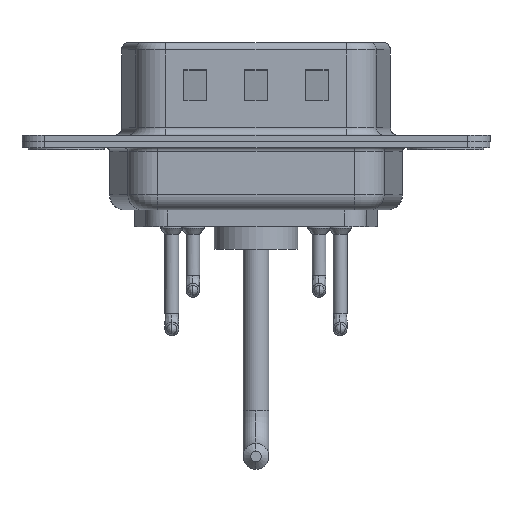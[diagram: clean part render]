
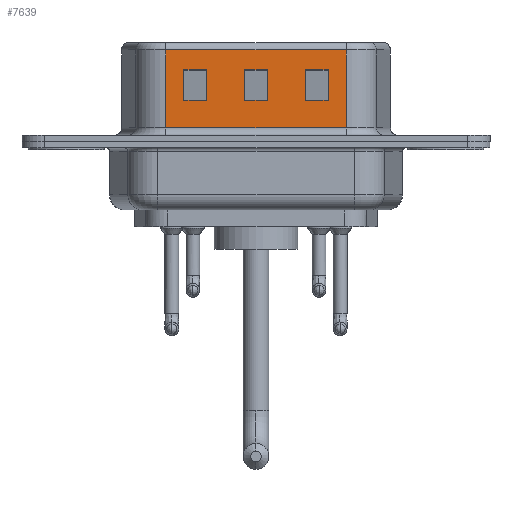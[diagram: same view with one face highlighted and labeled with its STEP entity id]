
A CAD part, front view. The second image highlights one B-rep face of the part: STEP entity #7639.
In plain terms, the highlighted planar face has unit normal (0, -1, 0).
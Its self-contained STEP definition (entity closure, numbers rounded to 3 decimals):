
#129 = ORIENTED_EDGE ( 'NONE', *, *, #16119, .T. ) ;
#251 = ORIENTED_EDGE ( 'NONE', *, *, #10598, .T. ) ;
#313 = CARTESIAN_POINT ( 'NONE',  ( 15.75, -4.55, 6.52 ) ) ;
#645 = VERTEX_POINT ( 'NONE', #16129 ) ;
#660 = CARTESIAN_POINT ( 'NONE',  ( 17.25, -4.55, 6.52 ) ) ;
#1310 = VERTEX_POINT ( 'NONE', #7896 ) ;
#1471 = DIRECTION ( 'NONE',  ( 1., 0., 0. ) ) ;
#1472 = EDGE_CURVE ( 'NONE', #3270, #1825, #12163, .T. ) ;
#1519 = LINE ( 'NONE', #12432, #11409 ) ;
#1825 = VERTEX_POINT ( 'NONE', #3703 ) ;
#1868 = VECTOR ( 'NONE', #4158, 1000. ) ;
#1922 = CARTESIAN_POINT ( 'NONE',  ( 18.451, -4.55, 6.02 ) ) ;
#2326 = VECTOR ( 'NONE', #16061, 1000. ) ;
#2384 = CARTESIAN_POINT ( 'NONE',  ( 7.75, -4.55, 4.705 ) ) ;
#2574 = CARTESIAN_POINT ( 'NONE',  ( 18.451, -4.55, 2.705 ) ) ;
#2583 = AXIS2_PLACEMENT_3D ( 'NONE', #14871, #13465, #9358 ) ;
#2734 = CARTESIAN_POINT ( 'NONE',  ( 9.25, -4.55, 6.52 ) ) ;
#2764 = DIRECTION ( 'NONE',  ( 0., 0., 1. ) ) ;
#3113 = DIRECTION ( 'NONE',  ( 1., 0., 0. ) ) ;
#3270 = VERTEX_POINT ( 'NONE', #14384 ) ;
#3328 = ORIENTED_EDGE ( 'NONE', *, *, #5694, .T. ) ;
#3396 = CARTESIAN_POINT ( 'NONE',  ( 7.75, -4.55, 6.52 ) ) ;
#3569 = VERTEX_POINT ( 'NONE', #11280 ) ;
#3645 = VECTOR ( 'NONE', #3113, 1000. ) ;
#3667 = LINE ( 'NONE', #11515, #8011 ) ;
#3675 = DIRECTION ( 'NONE',  ( 1., 0., 0. ) ) ;
#3703 = CARTESIAN_POINT ( 'NONE',  ( 6.549, -4.55, 0.9 ) ) ;
#3888 = VERTEX_POINT ( 'NONE', #16723 ) ;
#3982 = CARTESIAN_POINT ( 'NONE',  ( 6.549, -4.55, 6.52 ) ) ;
#4158 = DIRECTION ( 'NONE',  ( 0., 0., -1. ) ) ;
#4174 = EDGE_CURVE ( 'NONE', #8038, #3888, #8515, .T. ) ;
#4346 = VERTEX_POINT ( 'NONE', #6138 ) ;
#4417 = EDGE_LOOP ( 'NONE', ( #129, #14806, #17262, #14542 ) ) ;
#4756 = DIRECTION ( 'NONE',  ( 0., 0., -1. ) ) ;
#4987 = DIRECTION ( 'NONE',  ( -1., 0., 0. ) ) ;
#4997 = LINE ( 'NONE', #3396, #13685 ) ;
#5080 = CARTESIAN_POINT ( 'NONE',  ( 11.75, -4.55, 4.705 ) ) ;
#5178 = ORIENTED_EDGE ( 'NONE', *, *, #10489, .T. ) ;
#5450 = VERTEX_POINT ( 'NONE', #13937 ) ;
#5522 = VECTOR ( 'NONE', #15369, 1000. ) ;
#5602 = ORIENTED_EDGE ( 'NONE', *, *, #13185, .T. ) ;
#5694 = EDGE_CURVE ( 'NONE', #8637, #4346, #8235, .T. ) ;
#5772 = EDGE_CURVE ( 'NONE', #5450, #6888, #9490, .T. ) ;
#5799 = CARTESIAN_POINT ( 'NONE',  ( 18.451, -4.55, 4.705 ) ) ;
#6076 = DIRECTION ( 'NONE',  ( 0., 0., -1. ) ) ;
#6138 = CARTESIAN_POINT ( 'NONE',  ( 15.75, -4.55, 2.705 ) ) ;
#6238 = DIRECTION ( 'NONE',  ( 0., 0., 1. ) ) ;
#6563 = CARTESIAN_POINT ( 'NONE',  ( 18.451, -4.55, 6.02 ) ) ;
#6572 = DIRECTION ( 'NONE',  ( -1., 0., 0. ) ) ;
#6747 = DIRECTION ( 'NONE',  ( -1., 0., 0. ) ) ;
#6888 = VERTEX_POINT ( 'NONE', #7188 ) ;
#7151 = CARTESIAN_POINT ( 'NONE',  ( 9.25, -4.55, 2.705 ) ) ;
#7188 = CARTESIAN_POINT ( 'NONE',  ( 11.75, -4.55, 2.705 ) ) ;
#7518 = VECTOR ( 'NONE', #1471, 1000. ) ;
#7639 = ADVANCED_FACE ( 'NONE', ( #14687, #17189, #16116, #10528 ), #10445, .F. ) ;
#7896 = CARTESIAN_POINT ( 'NONE',  ( 18.451, -4.55, 0.9 ) ) ;
#7949 = LINE ( 'NONE', #9545, #8849 ) ;
#8011 = VECTOR ( 'NONE', #4756, 1000. ) ;
#8038 = VERTEX_POINT ( 'NONE', #2384 ) ;
#8148 = LINE ( 'NONE', #6563, #2326 ) ;
#8235 = LINE ( 'NONE', #14642, #8899 ) ;
#8307 = DIRECTION ( 'NONE',  ( 0., 0., 1. ) ) ;
#8395 = LINE ( 'NONE', #313, #10600 ) ;
#8451 = VERTEX_POINT ( 'NONE', #9517 ) ;
#8515 = LINE ( 'NONE', #12521, #3645 ) ;
#8637 = VERTEX_POINT ( 'NONE', #14894 ) ;
#8666 = EDGE_CURVE ( 'NONE', #12347, #3270, #8148, .T. ) ;
#8849 = VECTOR ( 'NONE', #14960, 1000. ) ;
#8899 = VECTOR ( 'NONE', #6572, 1000. ) ;
#8920 = VECTOR ( 'NONE', #4987, 1000. ) ;
#9030 = VERTEX_POINT ( 'NONE', #14519 ) ;
#9043 = EDGE_CURVE ( 'NONE', #3569, #5450, #7949, .T. ) ;
#9329 = EDGE_CURVE ( 'NONE', #12347, #1310, #3667, .T. ) ;
#9358 = DIRECTION ( 'NONE',  ( -1., 0., 0. ) ) ;
#9490 = LINE ( 'NONE', #2574, #12028 ) ;
#9517 = CARTESIAN_POINT ( 'NONE',  ( 17.25, -4.55, 4.705 ) ) ;
#9545 = CARTESIAN_POINT ( 'NONE',  ( 13.25, -4.55, 6.52 ) ) ;
#9785 = LINE ( 'NONE', #5799, #5522 ) ;
#9838 = ORIENTED_EDGE ( 'NONE', *, *, #11123, .T. ) ;
#10173 = ORIENTED_EDGE ( 'NONE', *, *, #17363, .T. ) ;
#10226 = LINE ( 'NONE', #14307, #8920 ) ;
#10445 = PLANE ( 'NONE',  #2583 ) ;
#10489 = EDGE_CURVE ( 'NONE', #4346, #9030, #8395, .T. ) ;
#10528 = FACE_OUTER_BOUND ( 'NONE', #11313, .T. ) ;
#10530 = VERTEX_POINT ( 'NONE', #7151 ) ;
#10598 = EDGE_CURVE ( 'NONE', #1825, #1310, #11862, .T. ) ;
#10600 = VECTOR ( 'NONE', #8307, 1000. ) ;
#10975 = CARTESIAN_POINT ( 'NONE',  ( 22.451, -4.55, 4.705 ) ) ;
#11024 = EDGE_CURVE ( 'NONE', #645, #8038, #4997, .T. ) ;
#11123 = EDGE_CURVE ( 'NONE', #8451, #8637, #12812, .T. ) ;
#11211 = ORIENTED_EDGE ( 'NONE', *, *, #16668, .T. ) ;
#11230 = VERTEX_POINT ( 'NONE', #5080 ) ;
#11280 = CARTESIAN_POINT ( 'NONE',  ( 13.25, -4.55, 4.705 ) ) ;
#11313 = EDGE_LOOP ( 'NONE', ( #14668, #11610, #12537, #251 ) ) ;
#11409 = VECTOR ( 'NONE', #2764, 1000. ) ;
#11467 = VECTOR ( 'NONE', #14698, 1000. ) ;
#11515 = CARTESIAN_POINT ( 'NONE',  ( 18.451, -4.55, 6.52 ) ) ;
#11610 = ORIENTED_EDGE ( 'NONE', *, *, #8666, .T. ) ;
#11862 = LINE ( 'NONE', #14249, #15664 ) ;
#11961 = LINE ( 'NONE', #2734, #11467 ) ;
#12028 = VECTOR ( 'NONE', #6747, 1000. ) ;
#12163 = LINE ( 'NONE', #3982, #1868 ) ;
#12347 = VERTEX_POINT ( 'NONE', #1922 ) ;
#12432 = CARTESIAN_POINT ( 'NONE',  ( 11.75, -4.55, 6.52 ) ) ;
#12521 = CARTESIAN_POINT ( 'NONE',  ( 14.451, -4.55, 4.705 ) ) ;
#12537 = ORIENTED_EDGE ( 'NONE', *, *, #1472, .T. ) ;
#12622 = ORIENTED_EDGE ( 'NONE', *, *, #5772, .T. ) ;
#12812 = LINE ( 'NONE', #660, #15105 ) ;
#13185 = EDGE_CURVE ( 'NONE', #6888, #11230, #1519, .T. ) ;
#13370 = LINE ( 'NONE', #10975, #7518 ) ;
#13465 = DIRECTION ( 'NONE',  ( 0., 1., 0. ) ) ;
#13685 = VECTOR ( 'NONE', #6238, 1000. ) ;
#13937 = CARTESIAN_POINT ( 'NONE',  ( 13.25, -4.55, 2.705 ) ) ;
#14249 = CARTESIAN_POINT ( 'NONE',  ( 18.451, -4.55, 0.9 ) ) ;
#14307 = CARTESIAN_POINT ( 'NONE',  ( 14.451, -4.55, 2.705 ) ) ;
#14384 = CARTESIAN_POINT ( 'NONE',  ( 6.549, -4.55, 6.02 ) ) ;
#14519 = CARTESIAN_POINT ( 'NONE',  ( 15.75, -4.55, 4.705 ) ) ;
#14542 = ORIENTED_EDGE ( 'NONE', *, *, #4174, .T. ) ;
#14642 = CARTESIAN_POINT ( 'NONE',  ( 22.451, -4.55, 2.705 ) ) ;
#14668 = ORIENTED_EDGE ( 'NONE', *, *, #9329, .F. ) ;
#14687 = FACE_BOUND ( 'NONE', #4417, .T. ) ;
#14698 = DIRECTION ( 'NONE',  ( 0., 0., -1. ) ) ;
#14806 = ORIENTED_EDGE ( 'NONE', *, *, #16762, .T. ) ;
#14871 = CARTESIAN_POINT ( 'NONE',  ( 18.451, -4.55, 6.52 ) ) ;
#14872 = EDGE_LOOP ( 'NONE', ( #9838, #3328, #5178, #10173 ) ) ;
#14894 = CARTESIAN_POINT ( 'NONE',  ( 17.25, -4.55, 2.705 ) ) ;
#14960 = DIRECTION ( 'NONE',  ( 0., 0., -1. ) ) ;
#15105 = VECTOR ( 'NONE', #6076, 1000. ) ;
#15285 = ORIENTED_EDGE ( 'NONE', *, *, #9043, .T. ) ;
#15369 = DIRECTION ( 'NONE',  ( 1., 0., 0. ) ) ;
#15664 = VECTOR ( 'NONE', #3675, 1000. ) ;
#16061 = DIRECTION ( 'NONE',  ( -1., 0., 0. ) ) ;
#16116 = FACE_BOUND ( 'NONE', #16234, .T. ) ;
#16119 = EDGE_CURVE ( 'NONE', #3888, #10530, #11961, .T. ) ;
#16129 = CARTESIAN_POINT ( 'NONE',  ( 7.75, -4.55, 2.705 ) ) ;
#16234 = EDGE_LOOP ( 'NONE', ( #11211, #15285, #12622, #5602 ) ) ;
#16668 = EDGE_CURVE ( 'NONE', #11230, #3569, #9785, .T. ) ;
#16723 = CARTESIAN_POINT ( 'NONE',  ( 9.25, -4.55, 4.705 ) ) ;
#16762 = EDGE_CURVE ( 'NONE', #10530, #645, #10226, .T. ) ;
#17189 = FACE_BOUND ( 'NONE', #14872, .T. ) ;
#17262 = ORIENTED_EDGE ( 'NONE', *, *, #11024, .T. ) ;
#17363 = EDGE_CURVE ( 'NONE', #9030, #8451, #13370, .T. ) ;
